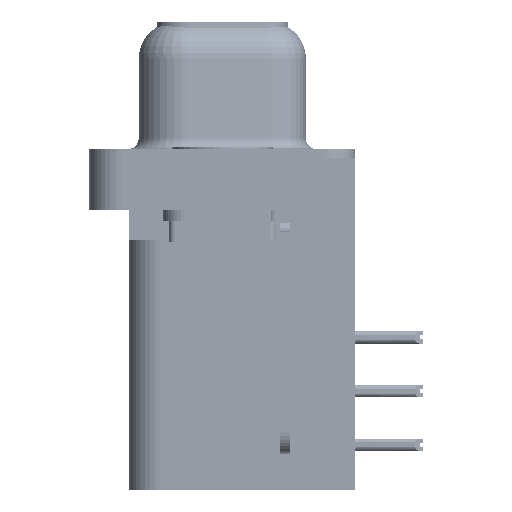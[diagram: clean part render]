
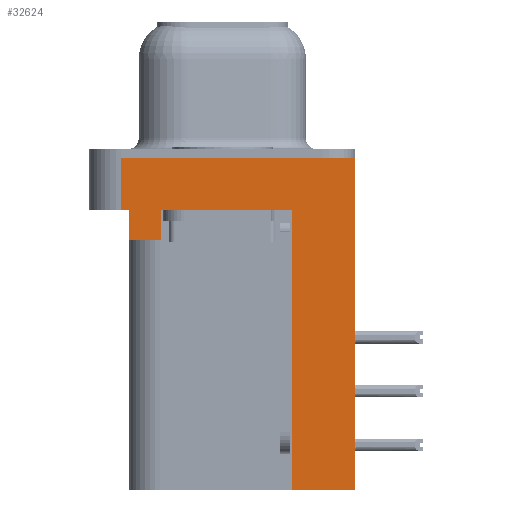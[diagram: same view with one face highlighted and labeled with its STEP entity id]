
A CAD part, left-side view. The second image highlights one B-rep face of the part: STEP entity #32624.
In plain terms, the highlighted planar face has unit normal (-1, 0, 0).
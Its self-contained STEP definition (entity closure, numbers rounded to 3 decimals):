
#85 = CARTESIAN_POINT ( 'NONE',  ( -2.91, -6.275, 0. ) ) ;
#399 = CARTESIAN_POINT ( 'NONE',  ( -2.91, -6.275, -2.5 ) ) ;
#425 = VECTOR ( 'NONE', #4286, 1000. ) ;
#1000 = EDGE_CURVE ( 'NONE', #29807, #25950, #13624, .T. ) ;
#1334 = VERTEX_POINT ( 'NONE', #50550 ) ;
#2039 = VECTOR ( 'NONE', #46559, 1000. ) ;
#3529 = LINE ( 'NONE', #45175, #43846 ) ;
#3654 = EDGE_CURVE ( 'NONE', #15487, #29807, #24193, .T. ) ;
#3690 = VERTEX_POINT ( 'NONE', #33356 ) ;
#4286 = DIRECTION ( 'NONE',  ( 0., -1., 0. ) ) ;
#4342 = DIRECTION ( 'NONE',  ( 0., 0., 1. ) ) ;
#4926 = VECTOR ( 'NONE', #41655, 1000. ) ;
#5172 = ORIENTED_EDGE ( 'NONE', *, *, #25850, .F. ) ;
#8072 = ORIENTED_EDGE ( 'NONE', *, *, #26797, .T. ) ;
#8291 = CARTESIAN_POINT ( 'NONE',  ( -2.91, 4.775, -2.5 ) ) ;
#9435 = VECTOR ( 'NONE', #15539, 1000. ) ;
#9808 = PLANE ( 'NONE',  #28267 ) ;
#10179 = EDGE_CURVE ( 'NONE', #1334, #3690, #10854, .T. ) ;
#10433 = ORIENTED_EDGE ( 'NONE', *, *, #10179, .T. ) ;
#10854 = LINE ( 'NONE', #31430, #40736 ) ;
#11451 = CARTESIAN_POINT ( 'NONE',  ( -2.91, -6.275, -2.5 ) ) ;
#11899 = VERTEX_POINT ( 'NONE', #27972 ) ;
#12110 = EDGE_CURVE ( 'NONE', #35576, #25950, #17616, .T. ) ;
#13624 = LINE ( 'NONE', #11451, #34224 ) ;
#13918 = EDGE_CURVE ( 'NONE', #41304, #11899, #3529, .T. ) ;
#14270 = DIRECTION ( 'NONE',  ( 0., 0., 1. ) ) ;
#15259 = VECTOR ( 'NONE', #14270, 1000. ) ;
#15487 = VERTEX_POINT ( 'NONE', #43837 ) ;
#15539 = DIRECTION ( 'NONE',  ( 0., -1., 0. ) ) ;
#17604 = DIRECTION ( 'NONE',  ( 0., 0., 1. ) ) ;
#17616 = LINE ( 'NONE', #29856, #4926 ) ;
#19579 = VERTEX_POINT ( 'NONE', #42178 ) ;
#19719 = EDGE_CURVE ( 'NONE', #11899, #3690, #39342, .T. ) ;
#20438 = LINE ( 'NONE', #40034, #41336 ) ;
#21591 = DIRECTION ( 'NONE',  ( 0., 0., 1. ) ) ;
#22812 = LINE ( 'NONE', #46309, #42559 ) ;
#24193 = LINE ( 'NONE', #34519, #15259 ) ;
#24628 = FACE_OUTER_BOUND ( 'NONE', #45552, .T. ) ;
#24696 = ORIENTED_EDGE ( 'NONE', *, *, #13918, .F. ) ;
#25191 = CARTESIAN_POINT ( 'NONE',  ( -2.91, 4.425, -2.5 ) ) ;
#25850 = EDGE_CURVE ( 'NONE', #19579, #46210, #22812, .T. ) ;
#25950 = VERTEX_POINT ( 'NONE', #34994 ) ;
#26775 = CARTESIAN_POINT ( 'NONE',  ( -2.91, -3.295, -15.7 ) ) ;
#26797 = EDGE_CURVE ( 'NONE', #41304, #46210, #41884, .T. ) ;
#27924 = ORIENTED_EDGE ( 'NONE', *, *, #32476, .F. ) ;
#27972 = CARTESIAN_POINT ( 'NONE',  ( -2.91, 4.775, 0. ) ) ;
#28267 = AXIS2_PLACEMENT_3D ( 'NONE', #37051, #41039, #17604 ) ;
#29807 = VERTEX_POINT ( 'NONE', #38048 ) ;
#29856 = CARTESIAN_POINT ( 'NONE',  ( -2.91, -3.295, -15.7 ) ) ;
#30525 = CARTESIAN_POINT ( 'NONE',  ( -2.91, -3.295, -15.7 ) ) ;
#31396 = ORIENTED_EDGE ( 'NONE', *, *, #47829, .F. ) ;
#31430 = CARTESIAN_POINT ( 'NONE',  ( -2.91, -6.275, -2.5 ) ) ;
#32476 = EDGE_CURVE ( 'NONE', #15487, #19579, #20438, .T. ) ;
#32624 = ADVANCED_FACE ( 'NONE', ( #24628 ), #9808, .T. ) ;
#33356 = CARTESIAN_POINT ( 'NONE',  ( -2.91, -6.275, 0. ) ) ;
#33573 = ORIENTED_EDGE ( 'NONE', *, *, #1000, .T. ) ;
#34224 = VECTOR ( 'NONE', #40560, 1000. ) ;
#34519 = CARTESIAN_POINT ( 'NONE',  ( -2.91, 2.895, -3.9 ) ) ;
#34994 = CARTESIAN_POINT ( 'NONE',  ( -2.91, -3.295, -2.5 ) ) ;
#35576 = VERTEX_POINT ( 'NONE', #30525 ) ;
#36019 = DIRECTION ( 'NONE',  ( 0., 1., 0. ) ) ;
#37051 = CARTESIAN_POINT ( 'NONE',  ( -2.91, -6.275, -2.5 ) ) ;
#37393 = ORIENTED_EDGE ( 'NONE', *, *, #12110, .F. ) ;
#38048 = CARTESIAN_POINT ( 'NONE',  ( -2.91, 2.895, -2.5 ) ) ;
#39342 = LINE ( 'NONE', #85, #9435 ) ;
#40034 = CARTESIAN_POINT ( 'NONE',  ( -2.91, 4.425, -3.9 ) ) ;
#40560 = DIRECTION ( 'NONE',  ( 0., -1., 0. ) ) ;
#40736 = VECTOR ( 'NONE', #4342, 1000. ) ;
#41039 = DIRECTION ( 'NONE',  ( -1., 0., 0. ) ) ;
#41304 = VERTEX_POINT ( 'NONE', #8291 ) ;
#41336 = VECTOR ( 'NONE', #36019, 1000. ) ;
#41655 = DIRECTION ( 'NONE',  ( 0., 0., 1. ) ) ;
#41884 = LINE ( 'NONE', #399, #425 ) ;
#42178 = CARTESIAN_POINT ( 'NONE',  ( -2.91, 4.425, -3.9 ) ) ;
#42303 = LINE ( 'NONE', #26775, #2039 ) ;
#42319 = DIRECTION ( 'NONE',  ( 0., 0., 1. ) ) ;
#42559 = VECTOR ( 'NONE', #42319, 1000. ) ;
#43837 = CARTESIAN_POINT ( 'NONE',  ( -2.91, 2.895, -3.9 ) ) ;
#43846 = VECTOR ( 'NONE', #21591, 1000. ) ;
#44302 = ORIENTED_EDGE ( 'NONE', *, *, #3654, .T. ) ;
#45175 = CARTESIAN_POINT ( 'NONE',  ( -2.91, 4.775, -2.5 ) ) ;
#45480 = ORIENTED_EDGE ( 'NONE', *, *, #19719, .F. ) ;
#45552 = EDGE_LOOP ( 'NONE', ( #45480, #24696, #8072, #5172, #27924, #44302, #33573, #37393, #31396, #10433 ) ) ;
#46210 = VERTEX_POINT ( 'NONE', #25191 ) ;
#46309 = CARTESIAN_POINT ( 'NONE',  ( -2.91, 4.425, -3.9 ) ) ;
#46559 = DIRECTION ( 'NONE',  ( 0., 1., 0. ) ) ;
#47829 = EDGE_CURVE ( 'NONE', #1334, #35576, #42303, .T. ) ;
#50550 = CARTESIAN_POINT ( 'NONE',  ( -2.91, -6.275, -15.7 ) ) ;
